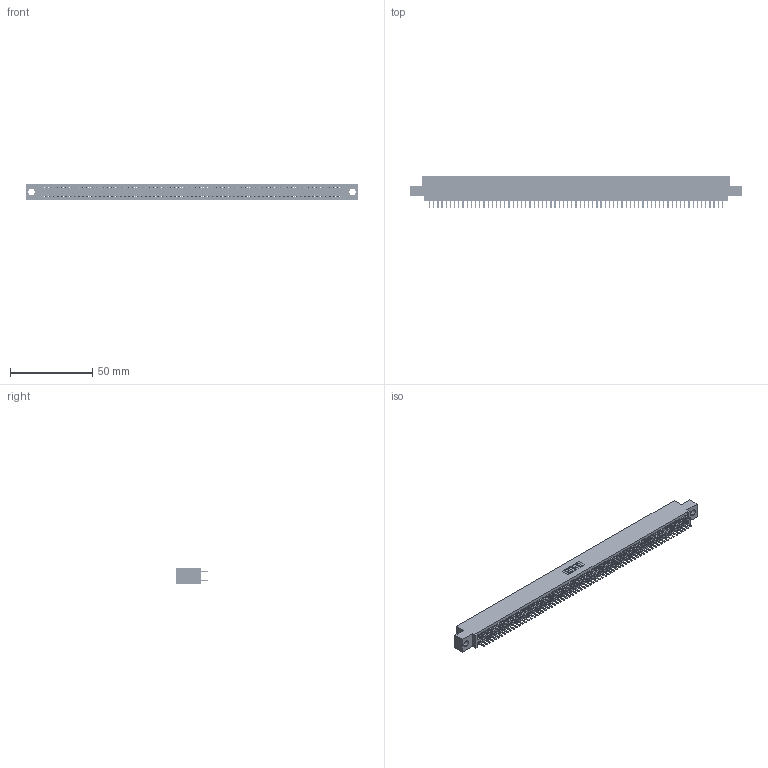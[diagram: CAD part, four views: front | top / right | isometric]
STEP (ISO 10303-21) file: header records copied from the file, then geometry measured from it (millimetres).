
FILE_DESCRIPTION (( 'STEP AP203' ), '1' );
FILE_NAME ('395-142-520-504.STEP', '2021-06-18T05:03:26', ( '' ), ( '' ), 'SwSTEP 2.0', 'SolidWorks 2020', '' );
FILE_SCHEMA (( 'CONFIG_CONTROL_DESIGN' ));
Length unit declared in the file: inch
Products named in the file (3): 345-292-001_345-293-120; 345 Part_0.110 Offset - 0.156 Dia-TI; 395-142-520-504
Assembly tree (143 placements, depth 2):
  395-142-520-504
    345 Part_0.110 Offset - 0.156 Dia-TI
    345-292-001_345-293-120  x142
Bounding box: 201.55 x 19.68 x 9.4 mm (x, y, z)
Volume: 19606.1 mm3; surface area: 29354.5 mm2
Topology: 143 solids, 143 shells, 7812 faces, 22683 edges, 14742 vertices
Faces by surface type: plane 5068, cylinder 2744
Entity records: 52469 total; most frequent: CARTESIAN_POINT 8786, ORIENTED_EDGE 8706, DIRECTION 7697, EDGE_CURVE 4353, LINE 3933, VECTOR 3933, VERTEX_POINT 2898, AXIS2_PLACEMENT_3D 1882
